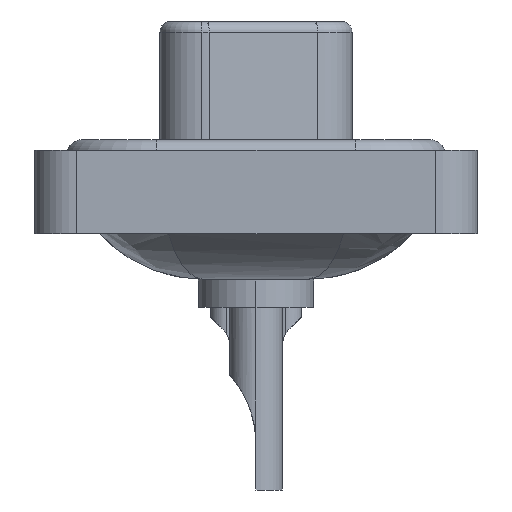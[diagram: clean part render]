
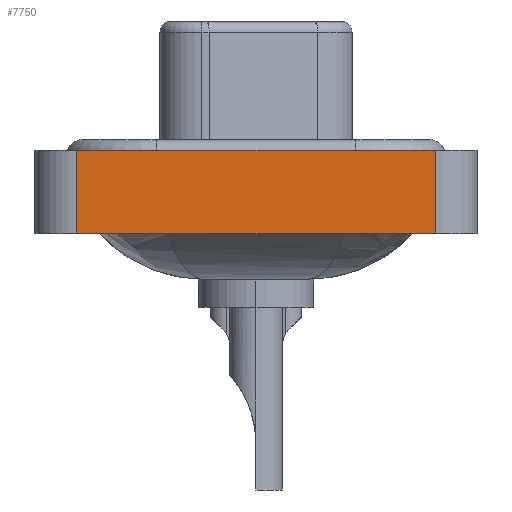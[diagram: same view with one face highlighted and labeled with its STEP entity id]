
A CAD part, left-side view. The second image highlights one B-rep face of the part: STEP entity #7750.
In plain terms, the highlighted planar face has unit normal (-1, 0, 0).
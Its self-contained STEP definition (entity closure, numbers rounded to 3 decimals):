
#1122 = CARTESIAN_POINT ( 'NONE',  ( -7.35, -8.55, -3.6 ) ) ;
#1338 = DIRECTION ( 'NONE',  ( 0., 0., 1. ) ) ;
#1654 = VERTEX_POINT ( 'NONE', #15177 ) ;
#2765 = DIRECTION ( 'NONE',  ( 0., 0., 1. ) ) ;
#3401 = ORIENTED_EDGE ( 'NONE', *, *, #14087, .F. ) ;
#3483 = VERTEX_POINT ( 'NONE', #1122 ) ;
#4227 = CARTESIAN_POINT ( 'NONE',  ( -7.35, 8.55, 0.4 ) ) ;
#4344 = DIRECTION ( 'NONE',  ( -1., 0., 0. ) ) ;
#4592 = LINE ( 'NONE', #6207, #14248 ) ;
#4714 = VECTOR ( 'NONE', #7132, 1000. ) ;
#5848 = CARTESIAN_POINT ( 'NONE',  ( -7.35, -8.55, -3.6 ) ) ;
#6024 = AXIS2_PLACEMENT_3D ( 'NONE', #5848, #4344, #2765 ) ;
#6207 = CARTESIAN_POINT ( 'NONE',  ( -7.35, -8.55, -3.6 ) ) ;
#6428 = ORIENTED_EDGE ( 'NONE', *, *, #16928, .T. ) ;
#7132 = DIRECTION ( 'NONE',  ( 0., -1., 0. ) ) ;
#7432 = FACE_OUTER_BOUND ( 'NONE', #16141, .T. ) ;
#7750 = ADVANCED_FACE ( 'NONE', ( #7432 ), #20449, .T. ) ;
#9731 = ORIENTED_EDGE ( 'NONE', *, *, #17202, .T. ) ;
#10848 = VECTOR ( 'NONE', #18221, 1000. ) ;
#11436 = CARTESIAN_POINT ( 'NONE',  ( -7.35, -8.55, 0.4 ) ) ;
#11952 = EDGE_CURVE ( 'NONE', #1654, #20333, #12537, .T. ) ;
#12264 = LINE ( 'NONE', #20021, #4714 ) ;
#12467 = ORIENTED_EDGE ( 'NONE', *, *, #11952, .F. ) ;
#12537 = LINE ( 'NONE', #12657, #17774 ) ;
#12657 = CARTESIAN_POINT ( 'NONE',  ( -7.35, 8.55, -3.6 ) ) ;
#13052 = LINE ( 'NONE', #11436, #10848 ) ;
#13141 = DIRECTION ( 'NONE',  ( 0., 0., 1. ) ) ;
#14087 = EDGE_CURVE ( 'NONE', #20333, #16884, #13052, .T. ) ;
#14248 = VECTOR ( 'NONE', #13141, 1000. ) ;
#15177 = CARTESIAN_POINT ( 'NONE',  ( -7.35, 8.55, -3.6 ) ) ;
#15889 = CARTESIAN_POINT ( 'NONE',  ( -7.35, -8.55, 0.4 ) ) ;
#16141 = EDGE_LOOP ( 'NONE', ( #6428, #3401, #12467, #9731 ) ) ;
#16884 = VERTEX_POINT ( 'NONE', #15889 ) ;
#16928 = EDGE_CURVE ( 'NONE', #3483, #16884, #4592, .T. ) ;
#17202 = EDGE_CURVE ( 'NONE', #1654, #3483, #12264, .T. ) ;
#17774 = VECTOR ( 'NONE', #1338, 1000. ) ;
#18221 = DIRECTION ( 'NONE',  ( 0., -1., 0. ) ) ;
#20021 = CARTESIAN_POINT ( 'NONE',  ( -7.35, -8.55, -3.6 ) ) ;
#20333 = VERTEX_POINT ( 'NONE', #4227 ) ;
#20449 = PLANE ( 'NONE',  #6024 ) ;
